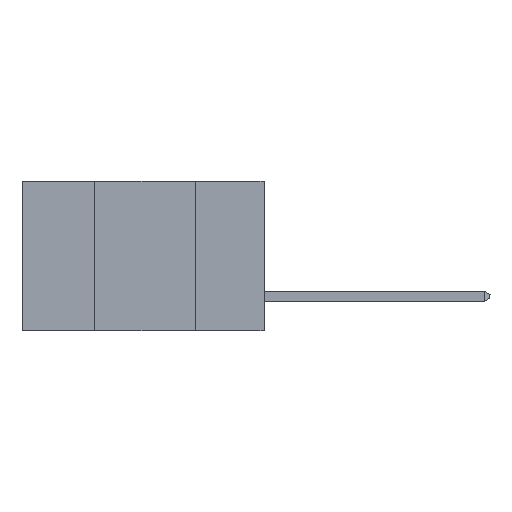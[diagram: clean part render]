
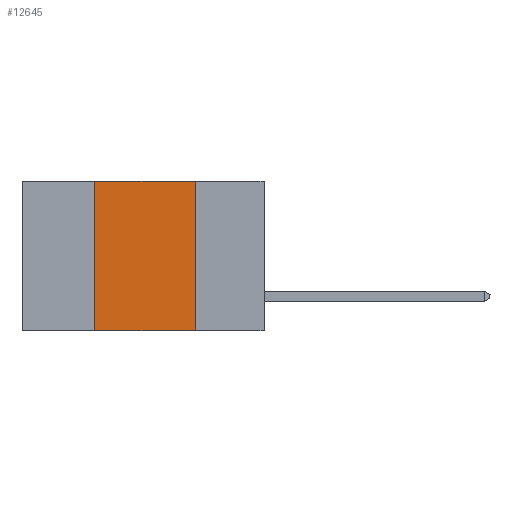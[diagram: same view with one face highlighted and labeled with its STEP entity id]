
A CAD part, left-side view. The second image highlights one B-rep face of the part: STEP entity #12645.
In plain terms, the highlighted planar face has unit normal (-1, 0, 0).
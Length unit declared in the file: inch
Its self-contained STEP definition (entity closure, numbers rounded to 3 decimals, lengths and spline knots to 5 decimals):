
#17 = VECTOR ( 'NONE', #229, 39.37008 ) ;
#229 = DIRECTION ( 'NONE',  ( 0., 0., 1. ) ) ;
#481 = EDGE_CURVE ( 'NONE', #9433, #3222, #4885, .T. ) ;
#504 = ORIENTED_EDGE ( 'NONE', *, *, #481, .F. ) ;
#878 = VECTOR ( 'NONE', #4840, 39.37008 ) ;
#1014 = AXIS2_PLACEMENT_3D ( 'NONE', #11022, #11120, #8079 ) ;
#1022 = EDGE_LOOP ( 'NONE', ( #3228, #1389, #504, #8609 ) ) ;
#1389 = ORIENTED_EDGE ( 'NONE', *, *, #2512, .F. ) ;
#2512 = EDGE_CURVE ( 'NONE', #3222, #5822, #8993, .T. ) ;
#3133 = PLANE ( 'NONE',  #1014 ) ;
#3222 = VERTEX_POINT ( 'NONE', #9249 ) ;
#3228 = ORIENTED_EDGE ( 'NONE', *, *, #6674, .F. ) ;
#3468 = EDGE_CURVE ( 'NONE', #9433, #8602, #10716, .T. ) ;
#3580 = CARTESIAN_POINT ( 'NONE',  ( 0., 0.17, 0. ) ) ;
#4266 = CARTESIAN_POINT ( 'NONE',  ( 0., 0.42, -0.37 ) ) ;
#4732 = CARTESIAN_POINT ( 'NONE',  ( 0., 0.6, 0. ) ) ;
#4840 = DIRECTION ( 'NONE',  ( 0., 0., -1. ) ) ;
#4885 = LINE ( 'NONE', #8161, #17 ) ;
#5451 = CARTESIAN_POINT ( 'NONE',  ( 0., 0.17, 0. ) ) ;
#5822 = VERTEX_POINT ( 'NONE', #5451 ) ;
#6275 = CARTESIAN_POINT ( 'NONE',  ( 0., 0.6, -0.37 ) ) ;
#6674 = EDGE_CURVE ( 'NONE', #5822, #8602, #10151, .T. ) ;
#7303 = DIRECTION ( 'NONE',  ( 0., -1., 0. ) ) ;
#7460 = CARTESIAN_POINT ( 'NONE',  ( 0., 0.17, -0.37 ) ) ;
#8079 = DIRECTION ( 'NONE',  ( 0., 0., -1. ) ) ;
#8161 = CARTESIAN_POINT ( 'NONE',  ( 0., 0.42, 0. ) ) ;
#8602 = VERTEX_POINT ( 'NONE', #7460 ) ;
#8609 = ORIENTED_EDGE ( 'NONE', *, *, #3468, .T. ) ;
#8993 = LINE ( 'NONE', #4732, #11049 ) ;
#9249 = CARTESIAN_POINT ( 'NONE',  ( 0., 0.42, 0. ) ) ;
#9433 = VERTEX_POINT ( 'NONE', #4266 ) ;
#10092 = VECTOR ( 'NONE', #7303, 39.37008 ) ;
#10151 = LINE ( 'NONE', #3580, #878 ) ;
#10380 = FACE_OUTER_BOUND ( 'NONE', #1022, .T. ) ;
#10665 = DIRECTION ( 'NONE',  ( 0., -1., 0. ) ) ;
#10716 = LINE ( 'NONE', #6275, #10092 ) ;
#11022 = CARTESIAN_POINT ( 'NONE',  ( 0., 0.6, 0. ) ) ;
#11049 = VECTOR ( 'NONE', #10665, 39.37008 ) ;
#11120 = DIRECTION ( 'NONE',  ( 1., 0., 0. ) ) ;
#12645 = ADVANCED_FACE ( 'NONE', ( #10380 ), #3133, .F. ) ;
